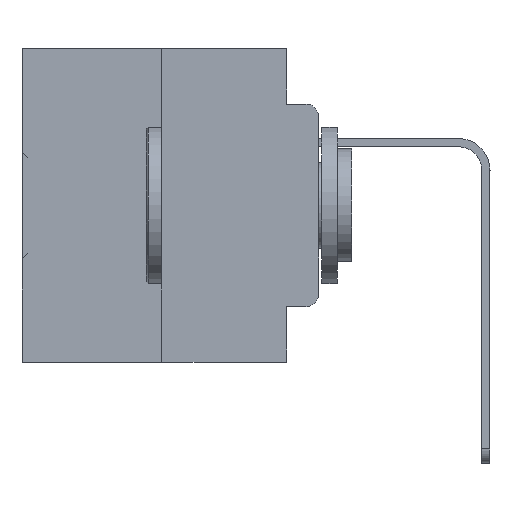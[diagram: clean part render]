
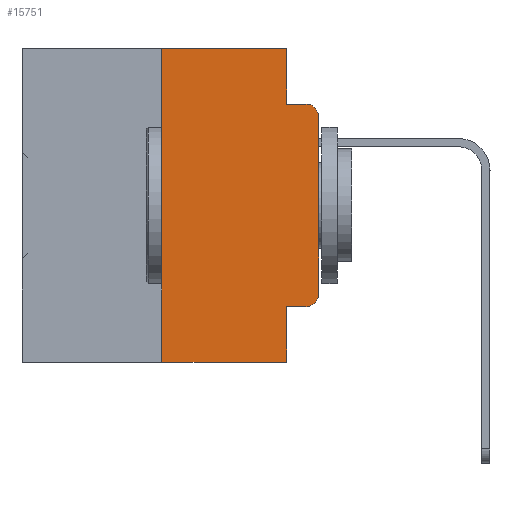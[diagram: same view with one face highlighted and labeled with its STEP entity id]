
A CAD part, left-side view. The second image highlights one B-rep face of the part: STEP entity #15751.
In plain terms, the highlighted planar face has unit normal (-1, 0, 0).
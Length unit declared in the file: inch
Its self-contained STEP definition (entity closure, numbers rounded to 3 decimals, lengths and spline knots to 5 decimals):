
#275 = DIRECTION ( 'NONE',  ( -1., 0., 0. ) ) ;
#556 = ORIENTED_EDGE ( 'NONE', *, *, #14844, .F. ) ;
#1717 = CIRCLE ( 'NONE', #28126, 0.02 ) ;
#1735 = EDGE_CURVE ( 'NONE', #24021, #21651, #27541, .T. ) ;
#1803 = CARTESIAN_POINT ( 'NONE',  ( 0., 0.051, -0.4115 ) ) ;
#1858 = LINE ( 'NONE', #12522, #22091 ) ;
#2677 = DIRECTION ( 'NONE',  ( 0., 0., 1. ) ) ;
#2976 = DIRECTION ( 'NONE',  ( 0., -1., 0. ) ) ;
#3130 = DIRECTION ( 'NONE',  ( 0., 0., -1. ) ) ;
#3363 = VERTEX_POINT ( 'NONE', #30066 ) ;
#4060 = DIRECTION ( 'NONE',  ( 0., -1., 0. ) ) ;
#5860 = DIRECTION ( 'NONE',  ( 0., -1., 0. ) ) ;
#7554 = PLANE ( 'NONE',  #25692 ) ;
#7638 = VECTOR ( 'NONE', #15626, 39.37008 ) ;
#7735 = CARTESIAN_POINT ( 'NONE',  ( 0., 0., -0.1085 ) ) ;
#8016 = VERTEX_POINT ( 'NONE', #23423 ) ;
#8044 = EDGE_CURVE ( 'NONE', #34067, #24021, #20454, .T. ) ;
#8559 = VERTEX_POINT ( 'NONE', #20807 ) ;
#9225 = ORIENTED_EDGE ( 'NONE', *, *, #1735, .T. ) ;
#9290 = AXIS2_PLACEMENT_3D ( 'NONE', #12192, #35066, #18121 ) ;
#10149 = DIRECTION ( 'NONE',  ( 1., 0., 0. ) ) ;
#10443 = LINE ( 'NONE', #25549, #24559 ) ;
#11076 = ORIENTED_EDGE ( 'NONE', *, *, #23027, .T. ) ;
#11098 = CARTESIAN_POINT ( 'NONE',  ( 0., 0.051, 0. ) ) ;
#11337 = DIRECTION ( 'NONE',  ( 0., 0., -1. ) ) ;
#12192 = CARTESIAN_POINT ( 'NONE',  ( 0., 0.02, -0.3915 ) ) ;
#12522 = CARTESIAN_POINT ( 'NONE',  ( 0., 0.473, 0. ) ) ;
#12741 = VERTEX_POINT ( 'NONE', #20357 ) ;
#12831 = DIRECTION ( 'NONE',  ( 0., 0., 1. ) ) ;
#14844 = EDGE_CURVE ( 'NONE', #3363, #20306, #1858, .T. ) ;
#15106 = LINE ( 'NONE', #32823, #7638 ) ;
#15626 = DIRECTION ( 'NONE',  ( 0., -1., 0. ) ) ;
#15751 = ADVANCED_FACE ( 'NONE', ( #30814 ), #7554, .F. ) ;
#15760 = VERTEX_POINT ( 'NONE', #1803 ) ;
#15892 = ORIENTED_EDGE ( 'NONE', *, *, #23215, .F. ) ;
#16969 = ORIENTED_EDGE ( 'NONE', *, *, #27627, .T. ) ;
#17244 = EDGE_CURVE ( 'NONE', #15760, #34067, #10443, .T. ) ;
#17427 = CARTESIAN_POINT ( 'NONE',  ( 0., 0.02, -0.0885 ) ) ;
#17738 = VECTOR ( 'NONE', #2976, 39.37008 ) ;
#18121 = DIRECTION ( 'NONE',  ( 0., 0., -1. ) ) ;
#18147 = LINE ( 'NONE', #25438, #23458 ) ;
#18687 = LINE ( 'NONE', #35692, #20894 ) ;
#20127 = VECTOR ( 'NONE', #2677, 39.37008 ) ;
#20306 = VERTEX_POINT ( 'NONE', #29712 ) ;
#20357 = CARTESIAN_POINT ( 'NONE',  ( 0., 0.051, -0.5 ) ) ;
#20454 = CIRCLE ( 'NONE', #9290, 0.02 ) ;
#20807 = CARTESIAN_POINT ( 'NONE',  ( 0., 0.051, -0.0885 ) ) ;
#20894 = VECTOR ( 'NONE', #12831, 39.37008 ) ;
#21409 = ORIENTED_EDGE ( 'NONE', *, *, #8044, .T. ) ;
#21651 = VERTEX_POINT ( 'NONE', #7735 ) ;
#22091 = VECTOR ( 'NONE', #4060, 39.37008 ) ;
#22515 = EDGE_CURVE ( 'NONE', #8016, #3363, #18687, .T. ) ;
#22879 = CARTESIAN_POINT ( 'NONE',  ( 0., 0.051, -0.0885 ) ) ;
#23027 = EDGE_CURVE ( 'NONE', #8016, #12741, #15106, .T. ) ;
#23215 = EDGE_CURVE ( 'NONE', #8559, #28567, #33139, .T. ) ;
#23423 = CARTESIAN_POINT ( 'NONE',  ( 0., 0.25, -0.5 ) ) ;
#23458 = VECTOR ( 'NONE', #30716, 39.37008 ) ;
#23912 = LINE ( 'NONE', #11098, #33125 ) ;
#24021 = VERTEX_POINT ( 'NONE', #28320 ) ;
#24559 = VECTOR ( 'NONE', #5860, 39.37008 ) ;
#25265 = ORIENTED_EDGE ( 'NONE', *, *, #34488, .F. ) ;
#25438 = CARTESIAN_POINT ( 'NONE',  ( 0., 0.051, 0. ) ) ;
#25549 = CARTESIAN_POINT ( 'NONE',  ( 0., 0.051, -0.4115 ) ) ;
#25692 = AXIS2_PLACEMENT_3D ( 'NONE', #32382, #10149, #30063 ) ;
#25889 = EDGE_CURVE ( 'NONE', #15760, #12741, #23912, .T. ) ;
#27541 = LINE ( 'NONE', #33261, #20127 ) ;
#27627 = EDGE_CURVE ( 'NONE', #21651, #28567, #1717, .T. ) ;
#28126 = AXIS2_PLACEMENT_3D ( 'NONE', #33838, #275, #3130 ) ;
#28320 = CARTESIAN_POINT ( 'NONE',  ( 0., 0., -0.3915 ) ) ;
#28567 = VERTEX_POINT ( 'NONE', #17427 ) ;
#29712 = CARTESIAN_POINT ( 'NONE',  ( 0., 0.051, 0. ) ) ;
#30063 = DIRECTION ( 'NONE',  ( 0., 0., -1. ) ) ;
#30066 = CARTESIAN_POINT ( 'NONE',  ( 0., 0.25, 0. ) ) ;
#30716 = DIRECTION ( 'NONE',  ( 0., 0., -1. ) ) ;
#30814 = FACE_OUTER_BOUND ( 'NONE', #32899, .T. ) ;
#31725 = ORIENTED_EDGE ( 'NONE', *, *, #22515, .F. ) ;
#32097 = CARTESIAN_POINT ( 'NONE',  ( 0., 0.02, -0.4115 ) ) ;
#32382 = CARTESIAN_POINT ( 'NONE',  ( 0., 0.473, 0. ) ) ;
#32683 = ORIENTED_EDGE ( 'NONE', *, *, #25889, .F. ) ;
#32823 = CARTESIAN_POINT ( 'NONE',  ( 0., 0.473, -0.5 ) ) ;
#32899 = EDGE_LOOP ( 'NONE', ( #9225, #16969, #15892, #25265, #556, #31725, #11076, #32683, #34335, #21409 ) ) ;
#33125 = VECTOR ( 'NONE', #11337, 39.37008 ) ;
#33139 = LINE ( 'NONE', #22879, #17738 ) ;
#33261 = CARTESIAN_POINT ( 'NONE',  ( 0., 0., 0. ) ) ;
#33838 = CARTESIAN_POINT ( 'NONE',  ( 0., 0.02, -0.1085 ) ) ;
#34067 = VERTEX_POINT ( 'NONE', #32097 ) ;
#34335 = ORIENTED_EDGE ( 'NONE', *, *, #17244, .T. ) ;
#34488 = EDGE_CURVE ( 'NONE', #20306, #8559, #18147, .T. ) ;
#35066 = DIRECTION ( 'NONE',  ( -1., 0., 0. ) ) ;
#35692 = CARTESIAN_POINT ( 'NONE',  ( 0., 0.25, 0. ) ) ;
